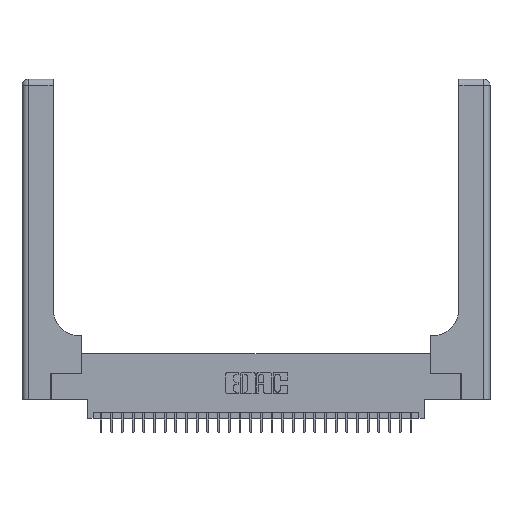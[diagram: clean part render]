
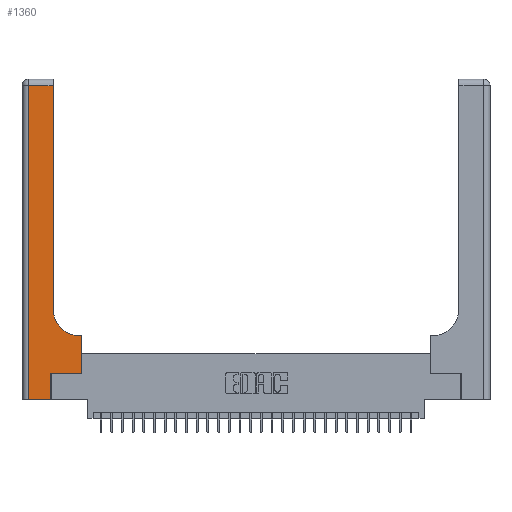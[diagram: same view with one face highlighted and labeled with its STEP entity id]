
A CAD part, top view. The second image highlights one B-rep face of the part: STEP entity #1360.
In plain terms, the highlighted planar face has unit normal (0, 0, 1).
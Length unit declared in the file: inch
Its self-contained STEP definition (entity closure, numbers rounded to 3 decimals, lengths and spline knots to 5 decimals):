
#403 = ORIENTED_EDGE ( 'NONE', *, *, #1002, .T. ) ;
#892 = DIRECTION ( 'NONE',  ( 1., 0., 0. ) ) ;
#1002 = EDGE_CURVE ( 'NONE', #4317, #6796, #6019, .T. ) ;
#1200 = ORIENTED_EDGE ( 'NONE', *, *, #10063, .T. ) ;
#1360 = ADVANCED_FACE ( 'NONE', ( #7537 ), #19299, .F. ) ;
#2007 = VECTOR ( 'NONE', #2959, 39.37008 ) ;
#2373 = VERTEX_POINT ( 'NONE', #10942 ) ;
#2449 = ORIENTED_EDGE ( 'NONE', *, *, #4333, .T. ) ;
#2530 = VECTOR ( 'NONE', #8468, 39.37008 ) ;
#2959 = DIRECTION ( 'NONE',  ( 1., 0., 0. ) ) ;
#2997 = VERTEX_POINT ( 'NONE', #16459 ) ;
#3221 = DIRECTION ( 'NONE',  ( -1., 0., 0. ) ) ;
#3576 = CARTESIAN_POINT ( 'NONE',  ( 0., 0., 0.37 ) ) ;
#3869 = LINE ( 'NONE', #3576, #4702 ) ;
#3965 = VERTEX_POINT ( 'NONE', #22834 ) ;
#4317 = VERTEX_POINT ( 'NONE', #19697 ) ;
#4333 = EDGE_CURVE ( 'NONE', #6796, #2373, #14440, .T. ) ;
#4702 = VECTOR ( 'NONE', #27060, 39.37008 ) ;
#5214 = DIRECTION ( 'NONE',  ( 0., 0., -1. ) ) ;
#5524 = DIRECTION ( 'NONE',  ( 0., 0., -1. ) ) ;
#6019 = LINE ( 'NONE', #27046, #8909 ) ;
#6416 = LINE ( 'NONE', #23122, #18758 ) ;
#6531 = LINE ( 'NONE', #25399, #8105 ) ;
#6795 = CARTESIAN_POINT ( 'NONE',  ( 0.06, 2.94, 0.37 ) ) ;
#6796 = VERTEX_POINT ( 'NONE', #6795 ) ;
#7133 = DIRECTION ( 'NONE',  ( 0., 1., 0. ) ) ;
#7147 = ORIENTED_EDGE ( 'NONE', *, *, #26159, .T. ) ;
#7537 = FACE_OUTER_BOUND ( 'NONE', #28293, .T. ) ;
#8087 = CARTESIAN_POINT ( 'NONE',  ( 0.06, 3., 0.37 ) ) ;
#8105 = VECTOR ( 'NONE', #7133, 39.37008 ) ;
#8468 = DIRECTION ( 'NONE',  ( 0., 1., 0. ) ) ;
#8909 = VECTOR ( 'NONE', #25192, 39.37008 ) ;
#9675 = CARTESIAN_POINT ( 'NONE',  ( 0.2915, 0.85, 0.37 ) ) ;
#9746 = CARTESIAN_POINT ( 'NONE',  ( 0.269, 0.25, 0.37 ) ) ;
#9827 = CIRCLE ( 'NONE', #21211, 0.25 ) ;
#10063 = EDGE_CURVE ( 'NONE', #2997, #22373, #9827, .T. ) ;
#10286 = VECTOR ( 'NONE', #22359, 39.37008 ) ;
#10942 = CARTESIAN_POINT ( 'NONE',  ( 0.06, 0., 0.37 ) ) ;
#11054 = DIRECTION ( 'NONE',  ( -1., 0., 0. ) ) ;
#12138 = ORIENTED_EDGE ( 'NONE', *, *, #16623, .T. ) ;
#12322 = CARTESIAN_POINT ( 'NONE',  ( 0.269, 0.25, 0.37 ) ) ;
#12491 = ORIENTED_EDGE ( 'NONE', *, *, #18312, .T. ) ;
#12910 = LINE ( 'NONE', #29462, #10286 ) ;
#13674 = VECTOR ( 'NONE', #19991, 39.37008 ) ;
#14440 = LINE ( 'NONE', #8087, #13674 ) ;
#14522 = VERTEX_POINT ( 'NONE', #28415 ) ;
#15810 = LINE ( 'NONE', #9746, #2007 ) ;
#16459 = CARTESIAN_POINT ( 'NONE',  ( 0.5415, 0.6, 0.37 ) ) ;
#16623 = EDGE_CURVE ( 'NONE', #14522, #3965, #6531, .T. ) ;
#16968 = CARTESIAN_POINT ( 'NONE',  ( 0., 3., 0.37 ) ) ;
#17890 = ORIENTED_EDGE ( 'NONE', *, *, #25480, .T. ) ;
#18312 = EDGE_CURVE ( 'NONE', #2373, #24193, #3869, .T. ) ;
#18506 = CARTESIAN_POINT ( 'NONE',  ( 0.269, 0., 0.37 ) ) ;
#18758 = VECTOR ( 'NONE', #11054, 39.37008 ) ;
#19299 = PLANE ( 'NONE',  #27521 ) ;
#19697 = CARTESIAN_POINT ( 'NONE',  ( 0.2915, 2.94, 0.37 ) ) ;
#19991 = DIRECTION ( 'NONE',  ( 0., -1., 0. ) ) ;
#20375 = LINE ( 'NONE', #18506, #2530 ) ;
#21211 = AXIS2_PLACEMENT_3D ( 'NONE', #26716, #5524, #892 ) ;
#22359 = DIRECTION ( 'NONE',  ( 0., 1., 0. ) ) ;
#22373 = VERTEX_POINT ( 'NONE', #9675 ) ;
#22834 = CARTESIAN_POINT ( 'NONE',  ( 0.5585, 0.6, 0.37 ) ) ;
#23122 = CARTESIAN_POINT ( 'NONE',  ( 0.2915, 0.6, 0.37 ) ) ;
#23601 = EDGE_CURVE ( 'NONE', #22373, #4317, #12910, .T. ) ;
#24193 = VERTEX_POINT ( 'NONE', #25539 ) ;
#24713 = VERTEX_POINT ( 'NONE', #12322 ) ;
#24920 = EDGE_CURVE ( 'NONE', #3965, #2997, #6416, .T. ) ;
#25192 = DIRECTION ( 'NONE',  ( -1., 0., 0. ) ) ;
#25399 = CARTESIAN_POINT ( 'NONE',  ( 0.5585, 0.25, 0.37 ) ) ;
#25480 = EDGE_CURVE ( 'NONE', #24713, #14522, #15810, .T. ) ;
#25539 = CARTESIAN_POINT ( 'NONE',  ( 0.269, 0., 0.37 ) ) ;
#26159 = EDGE_CURVE ( 'NONE', #24193, #24713, #20375, .T. ) ;
#26507 = ORIENTED_EDGE ( 'NONE', *, *, #23601, .T. ) ;
#26716 = CARTESIAN_POINT ( 'NONE',  ( 0.5415, 0.85, 0.37 ) ) ;
#27046 = CARTESIAN_POINT ( 'NONE',  ( 0., 2.94, 0.37 ) ) ;
#27060 = DIRECTION ( 'NONE',  ( 1., 0., 0. ) ) ;
#27121 = ORIENTED_EDGE ( 'NONE', *, *, #24920, .T. ) ;
#27521 = AXIS2_PLACEMENT_3D ( 'NONE', #16968, #5214, #3221 ) ;
#28293 = EDGE_LOOP ( 'NONE', ( #26507, #403, #2449, #12491, #7147, #17890, #12138, #27121, #1200 ) ) ;
#28415 = CARTESIAN_POINT ( 'NONE',  ( 0.5585, 0.25, 0.37 ) ) ;
#29462 = CARTESIAN_POINT ( 'NONE',  ( 0.2915, 3., 0.37 ) ) ;
